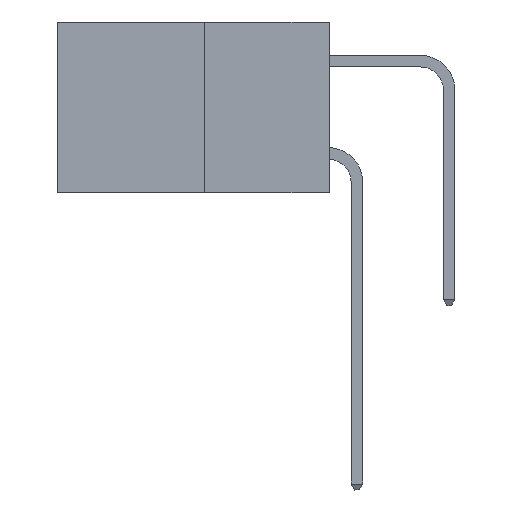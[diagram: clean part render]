
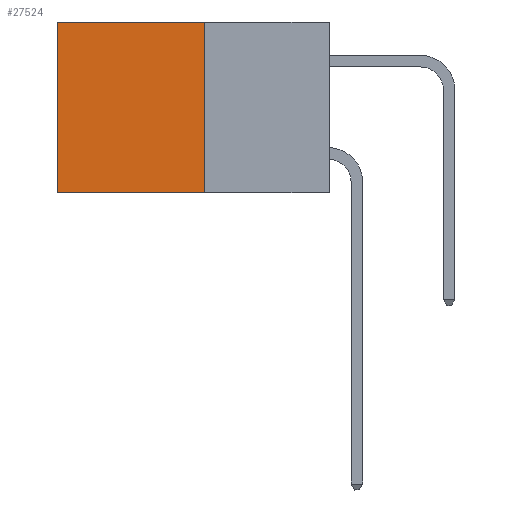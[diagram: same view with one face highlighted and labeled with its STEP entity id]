
A CAD part, left-side view. The second image highlights one B-rep face of the part: STEP entity #27524.
In plain terms, the highlighted planar face has unit normal (-1, 0, 0).
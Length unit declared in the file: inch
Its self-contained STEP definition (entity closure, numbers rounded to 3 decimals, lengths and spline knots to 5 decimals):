
#2073 = EDGE_LOOP ( 'NONE', ( #6642, #26537, #13480, #12753 ) ) ;
#3068 = PLANE ( 'NONE',  #9243 ) ;
#3296 = CARTESIAN_POINT ( 'NONE',  ( 0.277, 0.27, -0.37 ) ) ;
#5343 = LINE ( 'NONE', #17448, #11780 ) ;
#6539 = VERTEX_POINT ( 'NONE', #30160 ) ;
#6642 = ORIENTED_EDGE ( 'NONE', *, *, #22644, .T. ) ;
#8633 = CARTESIAN_POINT ( 'NONE',  ( 0.277, 0.27, -0.37 ) ) ;
#9007 = VERTEX_POINT ( 'NONE', #26880 ) ;
#9243 = AXIS2_PLACEMENT_3D ( 'NONE', #8633, #27369, #11368 ) ;
#10421 = LINE ( 'NONE', #32882, #30888 ) ;
#11368 = DIRECTION ( 'NONE',  ( 0., 0., -1. ) ) ;
#11780 = VECTOR ( 'NONE', #28123, 39.37008 ) ;
#12753 = ORIENTED_EDGE ( 'NONE', *, *, #18270, .T. ) ;
#13087 = VECTOR ( 'NONE', #19551, 39.37008 ) ;
#13480 = ORIENTED_EDGE ( 'NONE', *, *, #31774, .F. ) ;
#13683 = VECTOR ( 'NONE', #29834, 39.37008 ) ;
#14584 = CARTESIAN_POINT ( 'NONE',  ( 0.277, 0.59, 0. ) ) ;
#15499 = FACE_OUTER_BOUND ( 'NONE', #2073, .T. ) ;
#17448 = CARTESIAN_POINT ( 'NONE',  ( 0.277, 0.59, -0.37 ) ) ;
#18270 = EDGE_CURVE ( 'NONE', #9007, #27753, #10421, .T. ) ;
#19551 = DIRECTION ( 'NONE',  ( 0., 1., 0. ) ) ;
#20898 = VERTEX_POINT ( 'NONE', #21427 ) ;
#21427 = CARTESIAN_POINT ( 'NONE',  ( 0.277, 0.27, -0.37 ) ) ;
#22644 = EDGE_CURVE ( 'NONE', #27753, #6539, #5343, .T. ) ;
#25083 = EDGE_CURVE ( 'NONE', #20898, #6539, #27249, .T. ) ;
#26537 = ORIENTED_EDGE ( 'NONE', *, *, #25083, .F. ) ;
#26880 = CARTESIAN_POINT ( 'NONE',  ( 0.277, 0.27, 0. ) ) ;
#27148 = CARTESIAN_POINT ( 'NONE',  ( 0.277, 0.27, -0.37 ) ) ;
#27249 = LINE ( 'NONE', #3296, #13087 ) ;
#27369 = DIRECTION ( 'NONE',  ( 1., 0., 0. ) ) ;
#27524 = ADVANCED_FACE ( 'NONE', ( #15499 ), #3068, .F. ) ;
#27753 = VERTEX_POINT ( 'NONE', #14584 ) ;
#27841 = LINE ( 'NONE', #27148, #13683 ) ;
#28123 = DIRECTION ( 'NONE',  ( 0., 0., -1. ) ) ;
#29834 = DIRECTION ( 'NONE',  ( 0., 0., -1. ) ) ;
#30160 = CARTESIAN_POINT ( 'NONE',  ( 0.277, 0.59, -0.37 ) ) ;
#30209 = DIRECTION ( 'NONE',  ( 0., 1., 0. ) ) ;
#30888 = VECTOR ( 'NONE', #30209, 39.37008 ) ;
#31774 = EDGE_CURVE ( 'NONE', #9007, #20898, #27841, .T. ) ;
#32882 = CARTESIAN_POINT ( 'NONE',  ( 0.277, 0.27, 0. ) ) ;
